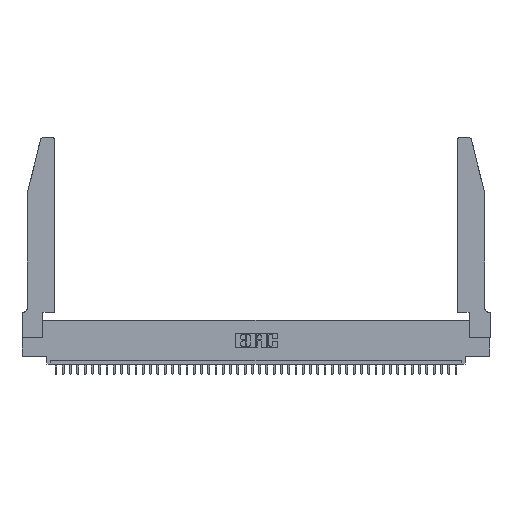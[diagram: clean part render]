
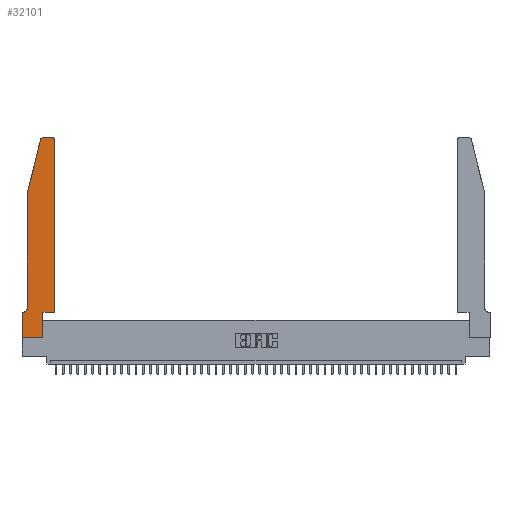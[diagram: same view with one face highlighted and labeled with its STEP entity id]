
A CAD part, top view. The second image highlights one B-rep face of the part: STEP entity #32101.
In plain terms, the highlighted planar face has unit normal (0, 0, 1).
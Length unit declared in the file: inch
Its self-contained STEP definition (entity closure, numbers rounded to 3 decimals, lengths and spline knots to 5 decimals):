
#210 = EDGE_CURVE ( 'NONE', #5844, #29435, #5616, .T. ) ;
#361 = VECTOR ( 'NONE', #35623, 39.37008 ) ;
#860 = DIRECTION ( 'NONE',  ( 0., 1., 0. ) ) ;
#1103 = ORIENTED_EDGE ( 'NONE', *, *, #37661, .T. ) ;
#1373 = VERTEX_POINT ( 'NONE', #36909 ) ;
#1596 = LINE ( 'NONE', #31089, #17914 ) ;
#1938 = CARTESIAN_POINT ( 'NONE',  ( 0., 0.35, 0.37 ) ) ;
#2436 = CARTESIAN_POINT ( 'NONE',  ( 0., 0., 0.37 ) ) ;
#3270 = CARTESIAN_POINT ( 'NONE',  ( 0.4505, 0.35, 0.37 ) ) ;
#3856 = EDGE_CURVE ( 'NONE', #37461, #24766, #18032, .T. ) ;
#4184 = CARTESIAN_POINT ( 'NONE',  ( 0.25487, 2.72718, 0.37 ) ) ;
#4284 = CARTESIAN_POINT ( 'NONE',  ( 0.4505, 0.35, 0.37 ) ) ;
#4818 = CARTESIAN_POINT ( 'NONE',  ( 0.2865, 0.35, 0.37 ) ) ;
#4833 = AXIS2_PLACEMENT_3D ( 'NONE', #20358, #30888, #41546 ) ;
#5616 = LINE ( 'NONE', #4284, #6220 ) ;
#5834 = AXIS2_PLACEMENT_3D ( 'NONE', #17531, #27319, #18068 ) ;
#5844 = VERTEX_POINT ( 'NONE', #29178 ) ;
#6220 = VECTOR ( 'NONE', #860, 39.37008 ) ;
#7652 = ORIENTED_EDGE ( 'NONE', *, *, #17680, .T. ) ;
#7799 = LINE ( 'NONE', #3270, #18096 ) ;
#8304 = CIRCLE ( 'NONE', #23730, 0.03 ) ;
#9189 = AXIS2_PLACEMENT_3D ( 'NONE', #29954, #19723, #19563 ) ;
#9283 = VERTEX_POINT ( 'NONE', #43510 ) ;
#9633 = CIRCLE ( 'NONE', #4833, 0.03 ) ;
#9668 = ORIENTED_EDGE ( 'NONE', *, *, #21974, .T. ) ;
#9812 = DIRECTION ( 'NONE',  ( 0., -1., 0. ) ) ;
#11059 = EDGE_CURVE ( 'NONE', #32974, #23108, #20268, .T. ) ;
#11869 = LINE ( 'NONE', #32764, #361 ) ;
#11993 = DIRECTION ( 'NONE',  ( 1., 0., 0. ) ) ;
#13631 = DIRECTION ( 'NONE',  ( 0., 0., 1. ) ) ;
#14210 = ORIENTED_EDGE ( 'NONE', *, *, #34664, .T. ) ;
#14667 = ORIENTED_EDGE ( 'NONE', *, *, #29789, .T. ) ;
#15026 = DIRECTION ( 'NONE',  ( -1., 0., 0. ) ) ;
#15926 = CARTESIAN_POINT ( 'NONE',  ( 0.0055, 0.35, 0.37 ) ) ;
#16499 = CARTESIAN_POINT ( 'NONE',  ( 0.284, 2.72, 0.37 ) ) ;
#17051 = LINE ( 'NONE', #2436, #25114 ) ;
#17531 = CARTESIAN_POINT ( 'NONE',  ( 0.0055, 0.42, 0.37 ) ) ;
#17680 = EDGE_CURVE ( 'NONE', #36810, #9283, #17051, .T. ) ;
#17802 = DIRECTION ( 'NONE',  ( 1., 0., 0. ) ) ;
#17914 = VECTOR ( 'NONE', #40977, 39.37008 ) ;
#18009 = VECTOR ( 'NONE', #15026, 39.37008 ) ;
#18032 = CIRCLE ( 'NONE', #5834, 0.07 ) ;
#18068 = DIRECTION ( 'NONE',  ( -1., 0., 0. ) ) ;
#18096 = VECTOR ( 'NONE', #17802, 39.37008 ) ;
#18661 = VERTEX_POINT ( 'NONE', #4818 ) ;
#19360 = DIRECTION ( 'NONE',  ( 0., -1., 0. ) ) ;
#19563 = DIRECTION ( 'NONE',  ( 1., 0., 0. ) ) ;
#19723 = DIRECTION ( 'NONE',  ( 0., 0., 1. ) ) ;
#20036 = VECTOR ( 'NONE', #22492, 39.37008 ) ;
#20253 = ORIENTED_EDGE ( 'NONE', *, *, #11059, .T. ) ;
#20268 = LINE ( 'NONE', #39526, #18009 ) ;
#20358 = CARTESIAN_POINT ( 'NONE',  ( 0.4205, 2.72, 0.37 ) ) ;
#21061 = CARTESIAN_POINT ( 'NONE',  ( 0.0755, 0.42, 0.37 ) ) ;
#21290 = CARTESIAN_POINT ( 'NONE',  ( 0.4205, 2.75, 0.37 ) ) ;
#21516 = EDGE_CURVE ( 'NONE', #42942, #37461, #41257, .T. ) ;
#21535 = VECTOR ( 'NONE', #19360, 39.37008 ) ;
#21672 = CARTESIAN_POINT ( 'NONE',  ( 0.0755, 2., 0.37 ) ) ;
#21677 = CARTESIAN_POINT ( 'NONE',  ( 0.4505, 2.72, 0.37 ) ) ;
#21974 = EDGE_CURVE ( 'NONE', #24766, #36810, #1596, .T. ) ;
#22193 = CARTESIAN_POINT ( 'NONE',  ( 0., 0., 0.37 ) ) ;
#22297 = FACE_OUTER_BOUND ( 'NONE', #34695, .T. ) ;
#22492 = DIRECTION ( 'NONE',  ( -0.239, -0.971, 0. ) ) ;
#23108 = VERTEX_POINT ( 'NONE', #43987 ) ;
#23664 = EDGE_CURVE ( 'NONE', #9283, #1373, #28737, .T. ) ;
#23730 = AXIS2_PLACEMENT_3D ( 'NONE', #16499, #13631, #44352 ) ;
#23742 = EDGE_CURVE ( 'NONE', #24516, #42942, #27124, .T. ) ;
#24492 = ORIENTED_EDGE ( 'NONE', *, *, #23664, .T. ) ;
#24516 = VERTEX_POINT ( 'NONE', #4184 ) ;
#24726 = EDGE_CURVE ( 'NONE', #29435, #32974, #9633, .T. ) ;
#24766 = VERTEX_POINT ( 'NONE', #15926 ) ;
#25114 = VECTOR ( 'NONE', #9812, 39.37008 ) ;
#25419 = ORIENTED_EDGE ( 'NONE', *, *, #21516, .T. ) ;
#26167 = ORIENTED_EDGE ( 'NONE', *, *, #210, .T. ) ;
#27124 = LINE ( 'NONE', #43381, #20036 ) ;
#27319 = DIRECTION ( 'NONE',  ( 0., 0., -1. ) ) ;
#28737 = LINE ( 'NONE', #22193, #41847 ) ;
#29178 = CARTESIAN_POINT ( 'NONE',  ( 0.4505, 0.35, 0.37 ) ) ;
#29435 = VERTEX_POINT ( 'NONE', #21677 ) ;
#29789 = EDGE_CURVE ( 'NONE', #23108, #24516, #8304, .T. ) ;
#29954 = CARTESIAN_POINT ( 'NONE',  ( 0., 0.35, 0.37 ) ) ;
#30888 = DIRECTION ( 'NONE',  ( 0., 0., 1. ) ) ;
#31089 = CARTESIAN_POINT ( 'NONE',  ( 0.0755, 0.35, 0.37 ) ) ;
#32101 = ADVANCED_FACE ( 'NONE', ( #22297 ), #33745, .T. ) ;
#32740 = ORIENTED_EDGE ( 'NONE', *, *, #23742, .T. ) ;
#32764 = CARTESIAN_POINT ( 'NONE',  ( 0.2865, 0.35, 0.37 ) ) ;
#32974 = VERTEX_POINT ( 'NONE', #21290 ) ;
#33745 = PLANE ( 'NONE',  #9189 ) ;
#34419 = ORIENTED_EDGE ( 'NONE', *, *, #3856, .T. ) ;
#34664 = EDGE_CURVE ( 'NONE', #18661, #5844, #7799, .T. ) ;
#34695 = EDGE_LOOP ( 'NONE', ( #20253, #14667, #32740, #25419, #34419, #9668, #7652, #24492, #1103, #14210, #26167, #37286 ) ) ;
#35623 = DIRECTION ( 'NONE',  ( 0., 1., 0. ) ) ;
#36810 = VERTEX_POINT ( 'NONE', #1938 ) ;
#36909 = CARTESIAN_POINT ( 'NONE',  ( 0.2865, 0., 0.37 ) ) ;
#37286 = ORIENTED_EDGE ( 'NONE', *, *, #24726, .T. ) ;
#37461 = VERTEX_POINT ( 'NONE', #21061 ) ;
#37661 = EDGE_CURVE ( 'NONE', #1373, #18661, #11869, .T. ) ;
#39526 = CARTESIAN_POINT ( 'NONE',  ( 0.2605, 2.75, 0.37 ) ) ;
#39924 = CARTESIAN_POINT ( 'NONE',  ( 0.0755, 2., 0.37 ) ) ;
#40977 = DIRECTION ( 'NONE',  ( -1., 0., 0. ) ) ;
#41257 = LINE ( 'NONE', #39924, #21535 ) ;
#41546 = DIRECTION ( 'NONE',  ( 1., 0., 0. ) ) ;
#41847 = VECTOR ( 'NONE', #11993, 39.37008 ) ;
#42942 = VERTEX_POINT ( 'NONE', #21672 ) ;
#43381 = CARTESIAN_POINT ( 'NONE',  ( 0.0755, 2., 0.37 ) ) ;
#43510 = CARTESIAN_POINT ( 'NONE',  ( 0., 0., 0.37 ) ) ;
#43987 = CARTESIAN_POINT ( 'NONE',  ( 0.284, 2.75, 0.37 ) ) ;
#44352 = DIRECTION ( 'NONE',  ( 1., 0., 0. ) ) ;
